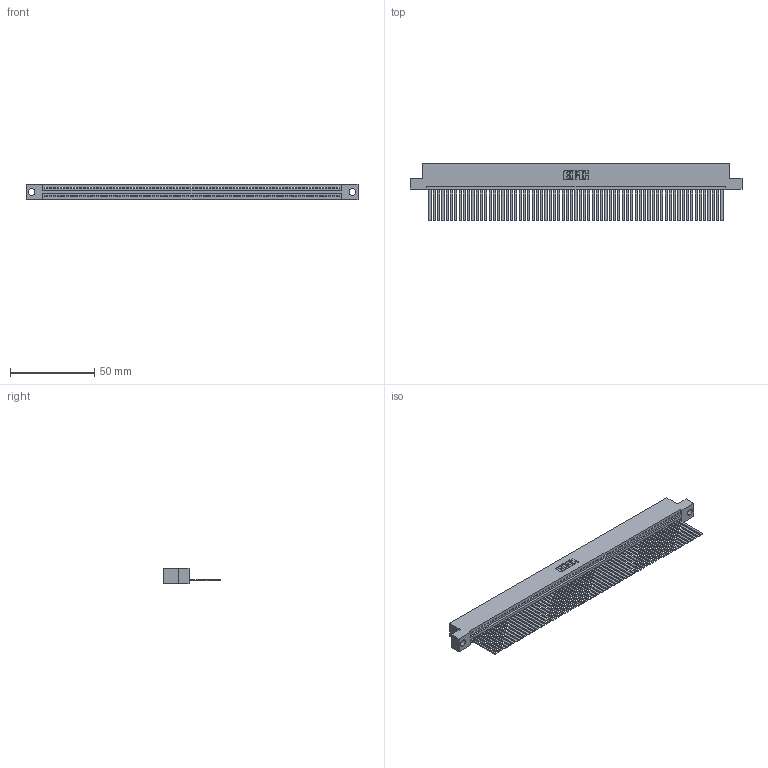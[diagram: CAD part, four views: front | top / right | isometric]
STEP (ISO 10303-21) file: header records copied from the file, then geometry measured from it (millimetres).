
FILE_DESCRIPTION (( 'STEP AP203' ), '1' );
FILE_NAME ('345-069-544-104.STEP', '2021-05-28T16:19:55', ( '' ), ( '' ), 'SwSTEP 2.0', 'SolidWorks 2020', '' );
FILE_SCHEMA (( 'CONFIG_CONTROL_DESIGN' ));
Products named in the file (3): 345 Part_Flush Mounting Lugs - 0.156 Dia-TI; 345-292-001_345-293-144; 345-069-544-104
Assembly tree (70 placements, depth 2):
  345-069-544-104
    345 Part_Flush Mounting Lugs - 0.156 Dia-TI
    345-292-001_345-293-144  x69
Bounding box: 196.47 x 33.96 x 9.4 mm (x, y, z)
Volume: 19575.2 mm3; surface area: 28622.1 mm2
Topology: 70 solids, 70 shells, 3728 faces, 11279 edges, 7426 vertices
Faces by surface type: plane 2578, cylinder 1150
Entity records: 48531 total; most frequent: ORIENTED_EDGE 8414, CARTESIAN_POINT 8413, DIRECTION 7305, EDGE_CURVE 4207, LINE 3803, VECTOR 3803, VERTEX_POINT 2802, AXIS2_PLACEMENT_3D 1751
